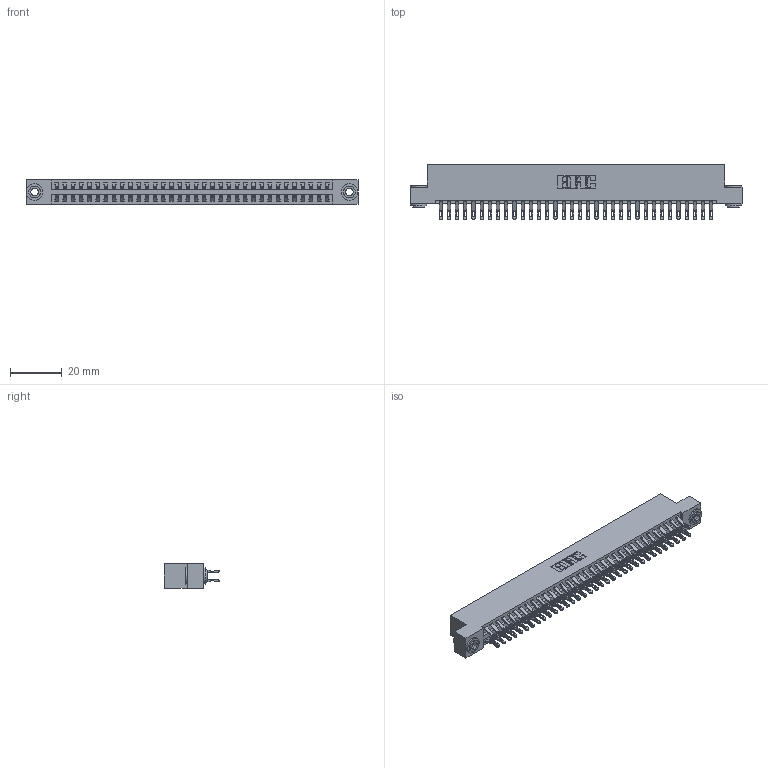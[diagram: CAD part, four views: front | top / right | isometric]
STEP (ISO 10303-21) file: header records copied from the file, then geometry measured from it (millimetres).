
FILE_DESCRIPTION (( 'STEP AP203' ), '1' );
FILE_NAME ('396-068-555-203.STEP', '2019-10-30T18:59:50', ( '' ), ( '' ), 'SwSTEP 2.0', 'SolidWorks 2016', '' );
FILE_SCHEMA (( 'CONFIG_CONTROL_DESIGN' ));
Length unit declared in the file: inch
Products named in the file (4): 345-250-002_345-250-002-102; 346 Part_Flush Mounting Lugs - 0.156 Dia-TH; 396-068-555-203; 345-292-001_555 Tail
Assembly tree (71 placements, depth 2):
  396-068-555-203
    346 Part_Flush Mounting Lugs - 0.156 Dia-TH
    345-292-001_555 Tail  x68
    345-250-002_345-250-002-102  x2
Bounding box: 128.52 x 21.46 x 9.4 mm (x, y, z)
Volume: 12687.2 mm3; surface area: 18230.9 mm2
Topology: 71 solids, 71 shells, 4104 faces, 12849 edges, 8562 vertices
Faces by surface type: plane 2330, cylinder 1766, cone 8
Entity records: 24242 total; most frequent: CARTESIAN_POINT 4017, ORIENTED_EDGE 3914, DIRECTION 3591, EDGE_CURVE 1957, LINE 1645, VECTOR 1645, VERTEX_POINT 1302, AXIS2_PLACEMENT_3D 973
